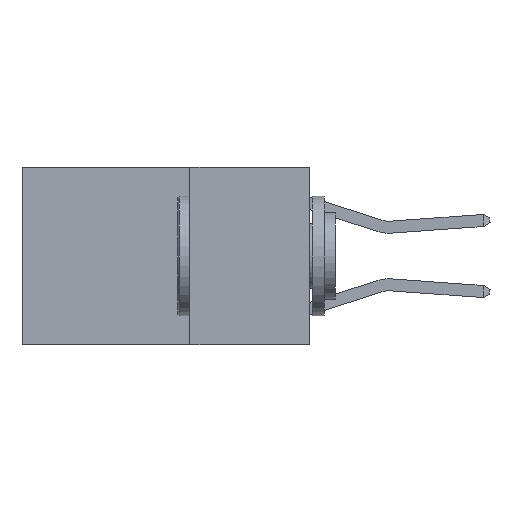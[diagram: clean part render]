
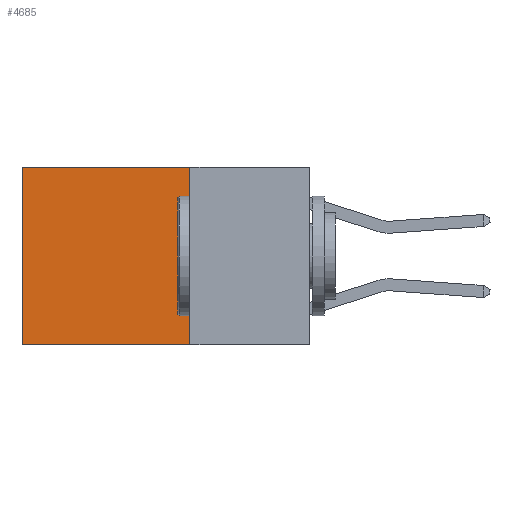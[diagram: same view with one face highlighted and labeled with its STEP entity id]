
A CAD part, left-side view. The second image highlights one B-rep face of the part: STEP entity #4685.
In plain terms, the highlighted planar face has unit normal (-1, 0, 0).
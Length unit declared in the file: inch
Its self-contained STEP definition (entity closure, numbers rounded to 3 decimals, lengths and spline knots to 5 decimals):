
#262 = EDGE_CURVE ( 'NONE', #11086, #3485, #9748, .T. ) ;
#374 = ORIENTED_EDGE ( 'NONE', *, *, #8480, .T. ) ;
#1035 = VERTEX_POINT ( 'NONE', #1360 ) ;
#1360 = CARTESIAN_POINT ( 'NONE',  ( 0.2625, 0.6, -0.37 ) ) ;
#1437 = EDGE_CURVE ( 'NONE', #10388, #1035, #11922, .T. ) ;
#1834 = DIRECTION ( 'NONE',  ( 0., 1., 0. ) ) ;
#1838 = CARTESIAN_POINT ( 'NONE',  ( 0.2625, 0.6, 0. ) ) ;
#2077 = EDGE_CURVE ( 'NONE', #3485, #1035, #2972, .T. ) ;
#2942 = FACE_OUTER_BOUND ( 'NONE', #8012, .T. ) ;
#2972 = LINE ( 'NONE', #9023, #5065 ) ;
#3485 = VERTEX_POINT ( 'NONE', #11215 ) ;
#4218 = CARTESIAN_POINT ( 'NONE',  ( 0.2625, 0.25, 0. ) ) ;
#4542 = DIRECTION ( 'NONE',  ( 0., 1., 0. ) ) ;
#4685 = ADVANCED_FACE ( 'NONE', ( #2942 ), #6657, .F. ) ;
#4851 = DIRECTION ( 'NONE',  ( 1., 0., 0. ) ) ;
#5065 = VECTOR ( 'NONE', #4542, 39.37008 ) ;
#5959 = CARTESIAN_POINT ( 'NONE',  ( 0.2625, 0.6, 0. ) ) ;
#6657 = PLANE ( 'NONE',  #11115 ) ;
#7084 = VECTOR ( 'NONE', #7888, 39.37008 ) ;
#7190 = CARTESIAN_POINT ( 'NONE',  ( 0.2625, 0.25, 0. ) ) ;
#7274 = ORIENTED_EDGE ( 'NONE', *, *, #2077, .F. ) ;
#7593 = DIRECTION ( 'NONE',  ( 0., 0., -1. ) ) ;
#7888 = DIRECTION ( 'NONE',  ( 0., 0., -1. ) ) ;
#8012 = EDGE_LOOP ( 'NONE', ( #10909, #7274, #8627, #374 ) ) ;
#8303 = VECTOR ( 'NONE', #7593, 39.37008 ) ;
#8480 = EDGE_CURVE ( 'NONE', #11086, #10388, #11918, .T. ) ;
#8534 = DIRECTION ( 'NONE',  ( 0., 0., -1. ) ) ;
#8599 = CARTESIAN_POINT ( 'NONE',  ( 0.2625, 0.25, 0. ) ) ;
#8627 = ORIENTED_EDGE ( 'NONE', *, *, #262, .F. ) ;
#9023 = CARTESIAN_POINT ( 'NONE',  ( 0.2625, 0.25, -0.37 ) ) ;
#9748 = LINE ( 'NONE', #4218, #7084 ) ;
#10358 = VECTOR ( 'NONE', #1834, 39.37008 ) ;
#10388 = VERTEX_POINT ( 'NONE', #5959 ) ;
#10909 = ORIENTED_EDGE ( 'NONE', *, *, #1437, .T. ) ;
#11086 = VERTEX_POINT ( 'NONE', #7190 ) ;
#11115 = AXIS2_PLACEMENT_3D ( 'NONE', #8599, #4851, #8534 ) ;
#11215 = CARTESIAN_POINT ( 'NONE',  ( 0.2625, 0.25, -0.37 ) ) ;
#11858 = CARTESIAN_POINT ( 'NONE',  ( 0.2625, 0.25, 0. ) ) ;
#11918 = LINE ( 'NONE', #11858, #10358 ) ;
#11922 = LINE ( 'NONE', #1838, #8303 ) ;
